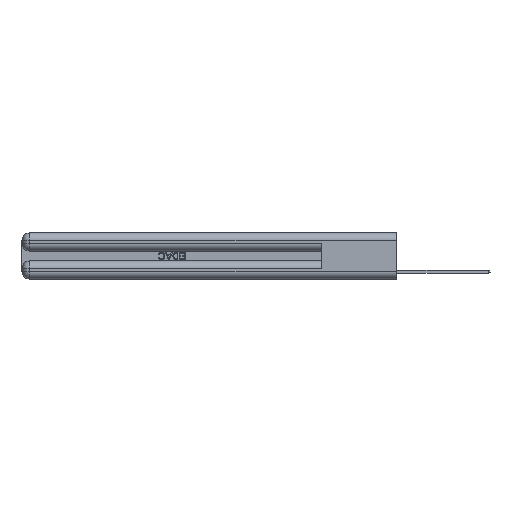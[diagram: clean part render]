
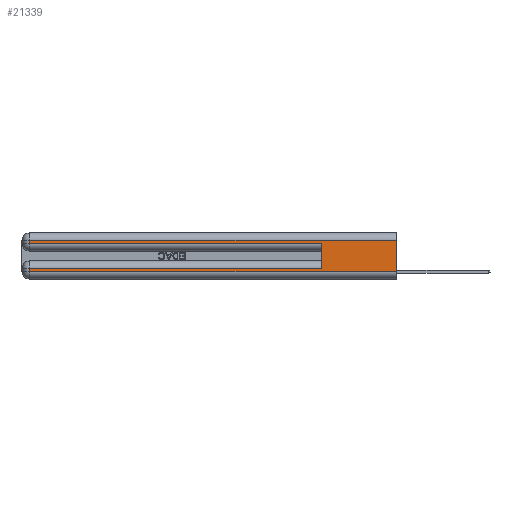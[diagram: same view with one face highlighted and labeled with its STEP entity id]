
A CAD part, left-side view. The second image highlights one B-rep face of the part: STEP entity #21339.
In plain terms, the highlighted planar face has unit normal (-1, 0, 0).
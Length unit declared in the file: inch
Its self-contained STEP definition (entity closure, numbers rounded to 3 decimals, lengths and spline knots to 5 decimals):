
#826 = CARTESIAN_POINT ( 'NONE',  ( 0., 0.6, 0.085 ) ) ;
#1793 = CARTESIAN_POINT ( 'NONE',  ( 0., 0.6, 0.285 ) ) ;
#1865 = VERTEX_POINT ( 'NONE', #29291 ) ;
#2921 = PLANE ( 'NONE',  #23942 ) ;
#2957 = VECTOR ( 'NONE', #13829, 39.37008 ) ;
#3274 = DIRECTION ( 'NONE',  ( 0., 0., -1. ) ) ;
#3467 = ORIENTED_EDGE ( 'NONE', *, *, #27068, .T. ) ;
#3698 = CARTESIAN_POINT ( 'NONE',  ( 0., 2.94, 0.37 ) ) ;
#4507 = ORIENTED_EDGE ( 'NONE', *, *, #8664, .T. ) ;
#4685 = CARTESIAN_POINT ( 'NONE',  ( 0., 0., 0.285 ) ) ;
#4949 = VECTOR ( 'NONE', #3274, 39.37008 ) ;
#5805 = DIRECTION ( 'NONE',  ( 0., 1., 0. ) ) ;
#5946 = VERTEX_POINT ( 'NONE', #13822 ) ;
#6224 = VECTOR ( 'NONE', #5805, 39.37008 ) ;
#6268 = VERTEX_POINT ( 'NONE', #28166 ) ;
#6601 = ORIENTED_EDGE ( 'NONE', *, *, #21044, .F. ) ;
#6798 = VERTEX_POINT ( 'NONE', #1793 ) ;
#7522 = CARTESIAN_POINT ( 'NONE',  ( 0., 2.94, 0.37 ) ) ;
#8664 = EDGE_CURVE ( 'NONE', #12065, #13800, #28822, .T. ) ;
#10340 = LINE ( 'NONE', #7522, #25457 ) ;
#10777 = CARTESIAN_POINT ( 'NONE',  ( 0., 0., 0.31 ) ) ;
#11344 = VERTEX_POINT ( 'NONE', #826 ) ;
#11425 = CARTESIAN_POINT ( 'NONE',  ( 0., 0.6, 0.145 ) ) ;
#12065 = VERTEX_POINT ( 'NONE', #15136 ) ;
#13279 = ORIENTED_EDGE ( 'NONE', *, *, #28229, .T. ) ;
#13456 = EDGE_CURVE ( 'NONE', #11344, #6798, #14554, .T. ) ;
#13522 = LINE ( 'NONE', #30399, #4949 ) ;
#13538 = CARTESIAN_POINT ( 'NONE',  ( 0., 2.94, 0.285 ) ) ;
#13628 = VECTOR ( 'NONE', #32051, 39.37008 ) ;
#13800 = VERTEX_POINT ( 'NONE', #13538 ) ;
#13822 = CARTESIAN_POINT ( 'NONE',  ( 0., 2.94, 0.06 ) ) ;
#13829 = DIRECTION ( 'NONE',  ( 0., 1., 0. ) ) ;
#14071 = LINE ( 'NONE', #16231, #13628 ) ;
#14554 = LINE ( 'NONE', #11425, #22510 ) ;
#15136 = CARTESIAN_POINT ( 'NONE',  ( 0., 2.94, 0.31 ) ) ;
#15501 = DIRECTION ( 'NONE',  ( 1., 0., 0. ) ) ;
#16231 = CARTESIAN_POINT ( 'NONE',  ( 0., 0., 0.06 ) ) ;
#17503 = EDGE_CURVE ( 'NONE', #32143, #5946, #10340, .T. ) ;
#17808 = CARTESIAN_POINT ( 'NONE',  ( 0., 0., 0.37 ) ) ;
#17817 = EDGE_CURVE ( 'NONE', #13800, #6798, #29800, .T. ) ;
#18082 = EDGE_LOOP ( 'NONE', ( #6601, #13279, #4507, #26717, #18410, #22167, #28018, #3467 ) ) ;
#18410 = ORIENTED_EDGE ( 'NONE', *, *, #13456, .F. ) ;
#19024 = DIRECTION ( 'NONE',  ( 0., 0., 1. ) ) ;
#19242 = DIRECTION ( 'NONE',  ( 0., 0., -1. ) ) ;
#21044 = EDGE_CURVE ( 'NONE', #1865, #6268, #13522, .T. ) ;
#21339 = ADVANCED_FACE ( 'NONE', ( #32508 ), #2921, .F. ) ;
#22167 = ORIENTED_EDGE ( 'NONE', *, *, #26062, .T. ) ;
#22510 = VECTOR ( 'NONE', #19024, 39.37008 ) ;
#22821 = VECTOR ( 'NONE', #27323, 39.37008 ) ;
#23942 = AXIS2_PLACEMENT_3D ( 'NONE', #17808, #15501, #30365 ) ;
#25457 = VECTOR ( 'NONE', #27868, 39.37008 ) ;
#25799 = LINE ( 'NONE', #10777, #6224 ) ;
#26062 = EDGE_CURVE ( 'NONE', #11344, #32143, #31496, .T. ) ;
#26717 = ORIENTED_EDGE ( 'NONE', *, *, #17817, .T. ) ;
#26716 = CARTESIAN_POINT ( 'NONE',  ( 0., 2.94, 0.085 ) ) ;
#27068 = EDGE_CURVE ( 'NONE', #5946, #6268, #14071, .T. ) ;
#27323 = DIRECTION ( 'NONE',  ( 0., -1., 0. ) ) ;
#27868 = DIRECTION ( 'NONE',  ( 0., 0., -1. ) ) ;
#28018 = ORIENTED_EDGE ( 'NONE', *, *, #17503, .T. ) ;
#28166 = CARTESIAN_POINT ( 'NONE',  ( 0., 0., 0.06 ) ) ;
#28211 = CARTESIAN_POINT ( 'NONE',  ( 0., 0., 0.085 ) ) ;
#28229 = EDGE_CURVE ( 'NONE', #1865, #12065, #25799, .T. ) ;
#28822 = LINE ( 'NONE', #3698, #31713 ) ;
#29291 = CARTESIAN_POINT ( 'NONE',  ( 0., 0., 0.31 ) ) ;
#29800 = LINE ( 'NONE', #4685, #22821 ) ;
#30365 = DIRECTION ( 'NONE',  ( 0., 0., -1. ) ) ;
#30399 = CARTESIAN_POINT ( 'NONE',  ( 0., 0., 0.37 ) ) ;
#31496 = LINE ( 'NONE', #28211, #2957 ) ;
#31713 = VECTOR ( 'NONE', #19242, 39.37008 ) ;
#32051 = DIRECTION ( 'NONE',  ( 0., -1., 0. ) ) ;
#32143 = VERTEX_POINT ( 'NONE', #26716 ) ;
#32508 = FACE_OUTER_BOUND ( 'NONE', #18082, .T. ) ;
